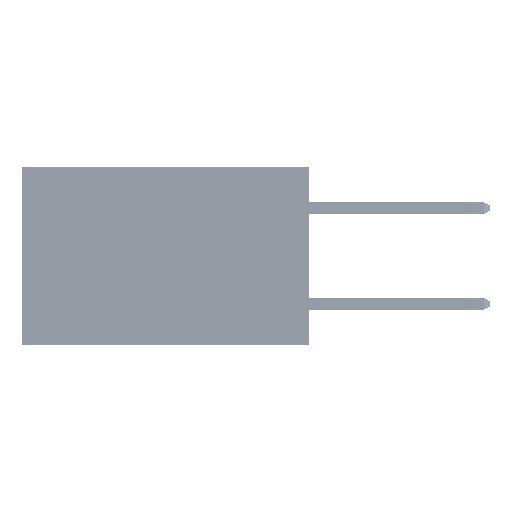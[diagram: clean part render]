
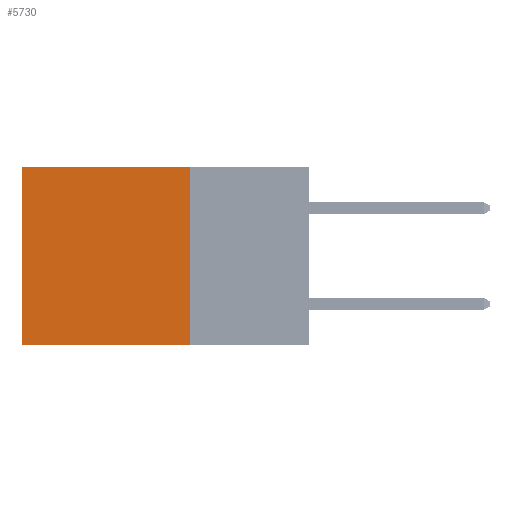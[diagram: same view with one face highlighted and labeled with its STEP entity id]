
A CAD part, left-side view. The second image highlights one B-rep face of the part: STEP entity #5730.
In plain terms, the highlighted planar face has unit normal (-1, 0, 0).
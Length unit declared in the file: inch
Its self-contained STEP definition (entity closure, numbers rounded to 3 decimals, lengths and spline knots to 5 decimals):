
#813 = VECTOR ( 'NONE', #12573, 39.37008 ) ;
#1783 = PLANE ( 'NONE',  #19299 ) ;
#3431 = ORIENTED_EDGE ( 'NONE', *, *, #4993, .T. ) ;
#4993 = EDGE_CURVE ( 'NONE', #12050, #11068, #42830, .T. ) ;
#5587 = VERTEX_POINT ( 'NONE', #43525 ) ;
#5730 = ADVANCED_FACE ( 'NONE', ( #38033 ), #1783, .F. ) ;
#5971 = CARTESIAN_POINT ( 'NONE',  ( 0.2875, 0.25, 0. ) ) ;
#6787 = DIRECTION ( 'NONE',  ( 1., 0., 0. ) ) ;
#6826 = DIRECTION ( 'NONE',  ( 0., 1., 0. ) ) ;
#8555 = CARTESIAN_POINT ( 'NONE',  ( 0.2875, 0.6, -0.37 ) ) ;
#11068 = VERTEX_POINT ( 'NONE', #8555 ) ;
#12050 = VERTEX_POINT ( 'NONE', #45359 ) ;
#12510 = EDGE_CURVE ( 'NONE', #44680, #5587, #27065, .T. ) ;
#12573 = DIRECTION ( 'NONE',  ( 0., 1., 0. ) ) ;
#13629 = CARTESIAN_POINT ( 'NONE',  ( 0.2875, 0.25, 0. ) ) ;
#14390 = ORIENTED_EDGE ( 'NONE', *, *, #23076, .F. ) ;
#14590 = LINE ( 'NONE', #19561, #813 ) ;
#16652 = VECTOR ( 'NONE', #6826, 39.37008 ) ;
#16718 = DIRECTION ( 'NONE',  ( 0., 0., -1. ) ) ;
#17038 = CARTESIAN_POINT ( 'NONE',  ( 0.2875, 0.6, 0. ) ) ;
#19181 = EDGE_LOOP ( 'NONE', ( #3431, #14390, #44005, #23178 ) ) ;
#19299 = AXIS2_PLACEMENT_3D ( 'NONE', #5971, #6787, #33578 ) ;
#19561 = CARTESIAN_POINT ( 'NONE',  ( 0.2875, 0.25, 0. ) ) ;
#21842 = CARTESIAN_POINT ( 'NONE',  ( 0.2875, 0.25, 0. ) ) ;
#23076 = EDGE_CURVE ( 'NONE', #5587, #11068, #24351, .T. ) ;
#23178 = ORIENTED_EDGE ( 'NONE', *, *, #32054, .T. ) ;
#24351 = LINE ( 'NONE', #25954, #16652 ) ;
#25954 = CARTESIAN_POINT ( 'NONE',  ( 0.2875, 0.25, -0.37 ) ) ;
#27065 = LINE ( 'NONE', #13629, #38342 ) ;
#32054 = EDGE_CURVE ( 'NONE', #44680, #12050, #14590, .T. ) ;
#32782 = VECTOR ( 'NONE', #16718, 39.37008 ) ;
#33578 = DIRECTION ( 'NONE',  ( 0., 0., -1. ) ) ;
#38033 = FACE_OUTER_BOUND ( 'NONE', #19181, .T. ) ;
#38342 = VECTOR ( 'NONE', #43829, 39.37008 ) ;
#42830 = LINE ( 'NONE', #17038, #32782 ) ;
#43525 = CARTESIAN_POINT ( 'NONE',  ( 0.2875, 0.25, -0.37 ) ) ;
#43829 = DIRECTION ( 'NONE',  ( 0., 0., -1. ) ) ;
#44005 = ORIENTED_EDGE ( 'NONE', *, *, #12510, .F. ) ;
#44680 = VERTEX_POINT ( 'NONE', #21842 ) ;
#45359 = CARTESIAN_POINT ( 'NONE',  ( 0.2875, 0.6, 0. ) ) ;
